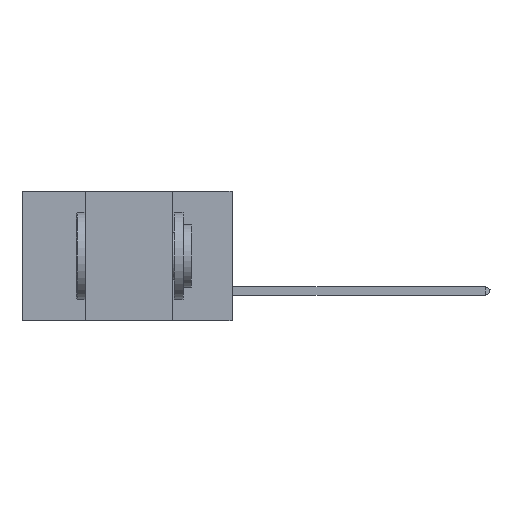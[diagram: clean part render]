
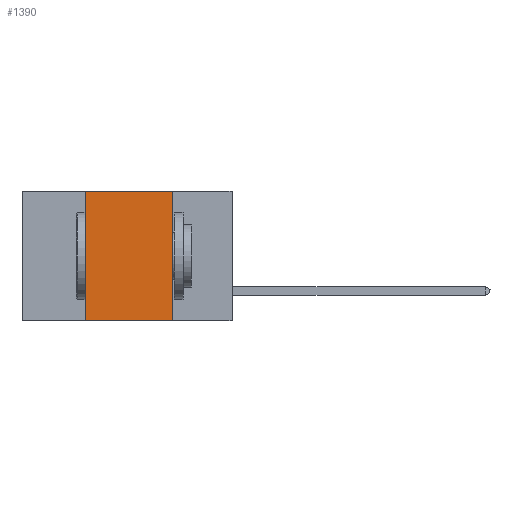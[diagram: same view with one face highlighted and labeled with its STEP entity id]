
A CAD part, left-side view. The second image highlights one B-rep face of the part: STEP entity #1390.
In plain terms, the highlighted planar face has unit normal (-1, 0, 0).
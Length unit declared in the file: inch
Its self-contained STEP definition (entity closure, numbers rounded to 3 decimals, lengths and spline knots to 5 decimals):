
#218 = VECTOR ( 'NONE', #30959, 39.37008 ) ;
#1390 = ADVANCED_FACE ( 'NONE', ( #36908 ), #31074, .F. ) ;
#1436 = AXIS2_PLACEMENT_3D ( 'NONE', #20444, #3673, #10730 ) ;
#3011 = VERTEX_POINT ( 'NONE', #28516 ) ;
#3673 = DIRECTION ( 'NONE',  ( 1., 0., 0. ) ) ;
#5431 = CARTESIAN_POINT ( 'NONE',  ( 0., 0.42, 0. ) ) ;
#5796 = CARTESIAN_POINT ( 'NONE',  ( 0., 0.6, 0. ) ) ;
#6274 = CARTESIAN_POINT ( 'NONE',  ( 0., 0.42, -0.37 ) ) ;
#7135 = VERTEX_POINT ( 'NONE', #20993 ) ;
#9537 = CARTESIAN_POINT ( 'NONE',  ( 0., 0.17, 0. ) ) ;
#9941 = EDGE_CURVE ( 'NONE', #18517, #3011, #10880, .T. ) ;
#10730 = DIRECTION ( 'NONE',  ( 0., 0., -1. ) ) ;
#10880 = LINE ( 'NONE', #40934, #27697 ) ;
#11077 = LINE ( 'NONE', #9537, #38921 ) ;
#12201 = DIRECTION ( 'NONE',  ( 0., 0., -1. ) ) ;
#15818 = DIRECTION ( 'NONE',  ( 0., -1., 0. ) ) ;
#18517 = VERTEX_POINT ( 'NONE', #6274 ) ;
#19713 = LINE ( 'NONE', #24660, #218 ) ;
#20444 = CARTESIAN_POINT ( 'NONE',  ( 0., 0.6, 0. ) ) ;
#20551 = EDGE_CURVE ( 'NONE', #18517, #20941, #19713, .T. ) ;
#20941 = VERTEX_POINT ( 'NONE', #5431 ) ;
#20993 = CARTESIAN_POINT ( 'NONE',  ( 0., 0.17, 0. ) ) ;
#21790 = EDGE_LOOP ( 'NONE', ( #31444, #36732, #40763, #29891 ) ) ;
#22917 = LINE ( 'NONE', #5796, #30699 ) ;
#24660 = CARTESIAN_POINT ( 'NONE',  ( 0., 0.42, 0. ) ) ;
#27697 = VECTOR ( 'NONE', #37692, 39.37008 ) ;
#28516 = CARTESIAN_POINT ( 'NONE',  ( 0., 0.17, -0.37 ) ) ;
#29891 = ORIENTED_EDGE ( 'NONE', *, *, #9941, .T. ) ;
#30699 = VECTOR ( 'NONE', #15818, 39.37008 ) ;
#30959 = DIRECTION ( 'NONE',  ( 0., 0., 1. ) ) ;
#31074 = PLANE ( 'NONE',  #1436 ) ;
#31444 = ORIENTED_EDGE ( 'NONE', *, *, #32593, .F. ) ;
#32593 = EDGE_CURVE ( 'NONE', #7135, #3011, #11077, .T. ) ;
#36657 = EDGE_CURVE ( 'NONE', #20941, #7135, #22917, .T. ) ;
#36732 = ORIENTED_EDGE ( 'NONE', *, *, #36657, .F. ) ;
#36908 = FACE_OUTER_BOUND ( 'NONE', #21790, .T. ) ;
#37692 = DIRECTION ( 'NONE',  ( 0., -1., 0. ) ) ;
#38921 = VECTOR ( 'NONE', #12201, 39.37008 ) ;
#40763 = ORIENTED_EDGE ( 'NONE', *, *, #20551, .F. ) ;
#40934 = CARTESIAN_POINT ( 'NONE',  ( 0., 0.6, -0.37 ) ) ;
